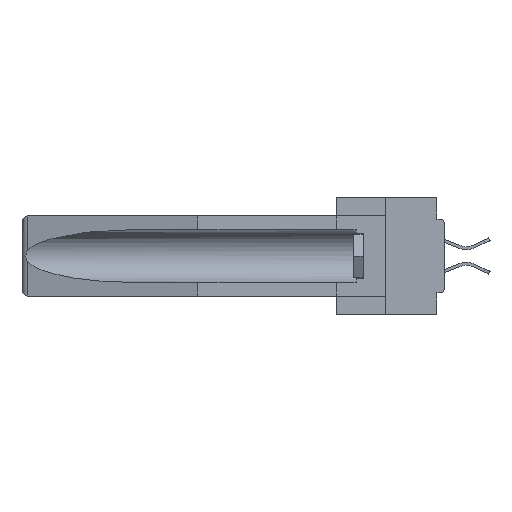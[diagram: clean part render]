
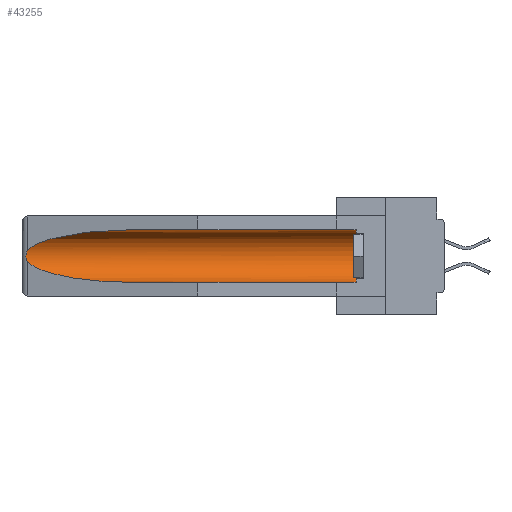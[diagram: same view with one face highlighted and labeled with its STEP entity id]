
A CAD part, left-side view. The second image highlights one B-rep face of the part: STEP entity #43255.
In plain terms, the highlighted cylindrical face has radius 2.857 mm (diameter 5.715 mm), a partial arc.
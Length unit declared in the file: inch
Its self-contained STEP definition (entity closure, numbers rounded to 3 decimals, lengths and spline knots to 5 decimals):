
#97 = DIRECTION ( 'NONE',  ( 0., 1., 0. ) ) ;
#1354 = CARTESIAN_POINT ( 'NONE',  ( 0.2673, 1.53269, -0.17917 ) ) ;
#2928 = CARTESIAN_POINT ( 'NONE',  ( 0.155, 1.07973, -0.284 ) ) ;
#3034 = CARTESIAN_POINT ( 'NONE',  ( 0.26537, 1.52718, -0.19328 ) ) ;
#5008 = CIRCLE ( 'NONE', #6485, 0.1125 ) ;
#5098 = EDGE_CURVE ( 'NONE', #38206, #45807, #5008, .T. ) ;
#5100 = CARTESIAN_POINT ( 'NONE',  ( 0.2675, 1.53308, -0.17534 ) ) ;
#5397 = EDGE_CURVE ( 'NONE', #38206, #18374, #8886, .T. ) ;
#5799 = ORIENTED_EDGE ( 'NONE', *, *, #22306, .T. ) ;
#6485 = AXIS2_PLACEMENT_3D ( 'NONE', #25093, #21378, #28374 ) ;
#8363 = VERTEX_POINT ( 'NONE', #3034 ) ;
#8886 = LINE ( 'NONE', #16297, #22792 ) ;
#9662 = ORIENTED_EDGE ( 'NONE', *, *, #33384, .T. ) ;
#9745 = CARTESIAN_POINT ( 'NONE',  ( 0.155, 1.07973, -0.284 ) ) ;
#10373 = B_SPLINE_CURVE_WITH_KNOTS ( 'NONE', 3,
 ( #19288, #33168, #43925, #22694, #44227, #5100, #1354, #25815, #29903, #15251 ),
 .UNSPECIFIED., .F., .F.,
 ( 4, 2, 2, 2, 4 ),
 ( 0., 0.00029, 0.00058, 0.00087, 0.00117 ),
 .UNSPECIFIED. ) ;
#11267 =( BOUNDED_CURVE ( )  B_SPLINE_CURVE ( 3, ( #16916, #38894, #17216, #9745 ),
 .UNSPECIFIED., .F., .F. ) 
 B_SPLINE_CURVE_WITH_KNOTS ( ( 4, 4 ),
 ( 0.1948, 1.5708 ),
 .UNSPECIFIED. ) 
 CURVE ( )  GEOMETRIC_REPRESENTATION_ITEM ( )  RATIONAL_B_SPLINE_CURVE ( ( 1., 0.848, 0.848, 1. ) ) 
 REPRESENTATION_ITEM ( '' )  );
#12357 = CARTESIAN_POINT ( 'NONE',  ( 0.155, 0.126, -0.059 ) ) ;
#12471 = EDGE_LOOP ( 'NONE', ( #28116, #9662, #5799, #34591, #44240, #30182 ) ) ;
#13270 = CARTESIAN_POINT ( 'NONE',  ( 0.26537, 1.52718, -0.14972 ) ) ;
#15251 = CARTESIAN_POINT ( 'NONE',  ( 0.26537, 1.52718, -0.19328 ) ) ;
#16297 = CARTESIAN_POINT ( 'NONE',  ( 0.155, -0.30754, -0.284 ) ) ;
#16916 = CARTESIAN_POINT ( 'NONE',  ( 0.26537, 1.52718, -0.19328 ) ) ;
#17216 = CARTESIAN_POINT ( 'NONE',  ( 0.21114, 1.30732, -0.284 ) ) ;
#17867 = CARTESIAN_POINT ( 'NONE',  ( 0.155, -0.30754, -0.1715 ) ) ;
#18374 = VERTEX_POINT ( 'NONE', #2928 ) ;
#18474 = LINE ( 'NONE', #27310, #22340 ) ;
#19288 = CARTESIAN_POINT ( 'NONE',  ( 0.26537, 1.52718, -0.14972 ) ) ;
#21378 = DIRECTION ( 'NONE',  ( 0., -1., 0. ) ) ;
#22306 = EDGE_CURVE ( 'NONE', #8363, #18374, #11267, .T. ) ;
#22340 = VECTOR ( 'NONE', #44814, 39.37008 ) ;
#22694 = CARTESIAN_POINT ( 'NONE',  ( 0.2673, 1.5327, -0.16383 ) ) ;
#22792 = VECTOR ( 'NONE', #27187, 39.37008 ) ;
#24136 = CARTESIAN_POINT ( 'NONE',  ( 0.26537, 1.52718, -0.14972 ) ) ;
#24368 = CARTESIAN_POINT ( 'NONE',  ( 0.25451, 1.48313, -0.09465 ) ) ;
#24948 =( BOUNDED_CURVE ( )  B_SPLINE_CURVE ( 3, ( #45141, #38559, #24368, #13270 ),
 .UNSPECIFIED., .F., .F. ) 
 B_SPLINE_CURVE_WITH_KNOTS ( ( 4, 4 ),
 ( 4.71239, 6.08839 ),
 .UNSPECIFIED. ) 
 CURVE ( )  GEOMETRIC_REPRESENTATION_ITEM ( )  RATIONAL_B_SPLINE_CURVE ( ( 1., 0.848, 0.848, 1. ) ) 
 REPRESENTATION_ITEM ( '' )  );
#25012 = DIRECTION ( 'NONE',  ( 0., 0., 1. ) ) ;
#25093 = CARTESIAN_POINT ( 'NONE',  ( 0.155, 0.126, -0.1715 ) ) ;
#25815 = CARTESIAN_POINT ( 'NONE',  ( 0.26655, 1.53094, -0.18657 ) ) ;
#27187 = DIRECTION ( 'NONE',  ( 0., 1., 0. ) ) ;
#27310 = CARTESIAN_POINT ( 'NONE',  ( 0.155, -0.30754, -0.059 ) ) ;
#28116 = ORIENTED_EDGE ( 'NONE', *, *, #41590, .T. ) ;
#28374 = DIRECTION ( 'NONE',  ( 0., 0., 1. ) ) ;
#28543 = VERTEX_POINT ( 'NONE', #28890 ) ;
#28890 = CARTESIAN_POINT ( 'NONE',  ( 0.155, 1.07973, -0.059 ) ) ;
#29903 = CARTESIAN_POINT ( 'NONE',  ( 0.26597, 1.5296, -0.19026 ) ) ;
#30182 = ORIENTED_EDGE ( 'NONE', *, *, #44905, .T. ) ;
#30876 = FACE_OUTER_BOUND ( 'NONE', #12471, .T. ) ;
#31250 = CARTESIAN_POINT ( 'NONE',  ( 0.155, 0.126, -0.284 ) ) ;
#33168 = CARTESIAN_POINT ( 'NONE',  ( 0.26597, 1.52961, -0.15275 ) ) ;
#33384 = EDGE_CURVE ( 'NONE', #41264, #8363, #10373, .T. ) ;
#34591 = ORIENTED_EDGE ( 'NONE', *, *, #5397, .F. ) ;
#38206 = VERTEX_POINT ( 'NONE', #31250 ) ;
#38559 = CARTESIAN_POINT ( 'NONE',  ( 0.21114, 1.30732, -0.059 ) ) ;
#38894 = CARTESIAN_POINT ( 'NONE',  ( 0.25451, 1.48313, -0.24835 ) ) ;
#39231 = CYLINDRICAL_SURFACE ( 'NONE', #45616, 0.1125 ) ;
#41264 = VERTEX_POINT ( 'NONE', #24136 ) ;
#41590 = EDGE_CURVE ( 'NONE', #28543, #41264, #24948, .T. ) ;
#43255 = ADVANCED_FACE ( 'NONE', ( #30876 ), #39231, .F. ) ;
#43925 = CARTESIAN_POINT ( 'NONE',  ( 0.26654, 1.53092, -0.15636 ) ) ;
#44227 = CARTESIAN_POINT ( 'NONE',  ( 0.2675, 1.53308, -0.16763 ) ) ;
#44240 = ORIENTED_EDGE ( 'NONE', *, *, #5098, .T. ) ;
#44814 = DIRECTION ( 'NONE',  ( 0., 1., 0. ) ) ;
#44905 = EDGE_CURVE ( 'NONE', #45807, #28543, #18474, .T. ) ;
#45141 = CARTESIAN_POINT ( 'NONE',  ( 0.155, 1.07973, -0.059 ) ) ;
#45616 = AXIS2_PLACEMENT_3D ( 'NONE', #17867, #97, #25012 ) ;
#45807 = VERTEX_POINT ( 'NONE', #12357 ) ;
